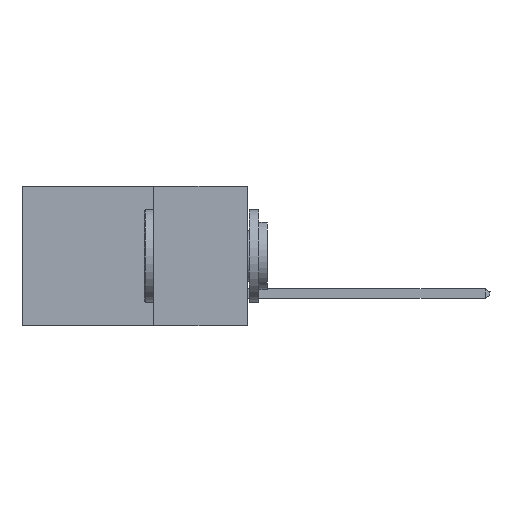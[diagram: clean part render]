
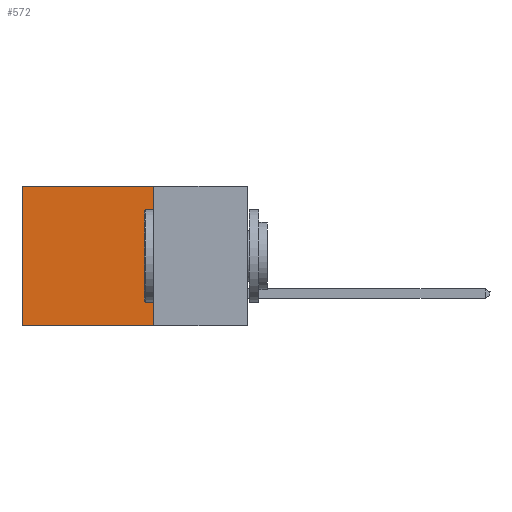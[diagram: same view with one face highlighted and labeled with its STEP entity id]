
A CAD part, left-side view. The second image highlights one B-rep face of the part: STEP entity #572.
In plain terms, the highlighted planar face has unit normal (-1, 0, 0).
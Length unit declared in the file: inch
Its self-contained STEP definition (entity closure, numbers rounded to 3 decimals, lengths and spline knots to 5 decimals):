
#572 = ADVANCED_FACE ( 'NONE', ( #11621 ), #6378, .F. ) ;
#764 = CARTESIAN_POINT ( 'NONE',  ( 0.2615, 0.6, -0.37 ) ) ;
#951 = ORIENTED_EDGE ( 'NONE', *, *, #10089, .F. ) ;
#1567 = VECTOR ( 'NONE', #8770, 39.37008 ) ;
#2288 = LINE ( 'NONE', #6314, #15878 ) ;
#3430 = VERTEX_POINT ( 'NONE', #7115 ) ;
#3524 = DIRECTION ( 'NONE',  ( 0., 1., 0. ) ) ;
#4733 = EDGE_CURVE ( 'NONE', #8559, #3430, #13982, .T. ) ;
#4832 = VERTEX_POINT ( 'NONE', #6330 ) ;
#5613 = VECTOR ( 'NONE', #9853, 39.37008 ) ;
#6314 = CARTESIAN_POINT ( 'NONE',  ( 0.2615, 0.25, -0.37 ) ) ;
#6330 = CARTESIAN_POINT ( 'NONE',  ( 0.2615, 0.25, 0. ) ) ;
#6378 = PLANE ( 'NONE',  #8142 ) ;
#6463 = ORIENTED_EDGE ( 'NONE', *, *, #14785, .T. ) ;
#6838 = CARTESIAN_POINT ( 'NONE',  ( 0.2615, 0.6, 0. ) ) ;
#6924 = ORIENTED_EDGE ( 'NONE', *, *, #4733, .T. ) ;
#7115 = CARTESIAN_POINT ( 'NONE',  ( 0.2615, 0.6, -0.37 ) ) ;
#8142 = AXIS2_PLACEMENT_3D ( 'NONE', #10039, #16994, #13084 ) ;
#8173 = VECTOR ( 'NONE', #14546, 39.37008 ) ;
#8559 = VERTEX_POINT ( 'NONE', #6838 ) ;
#8770 = DIRECTION ( 'NONE',  ( 0., 0., -1. ) ) ;
#9082 = LINE ( 'NONE', #10476, #8173 ) ;
#9273 = VERTEX_POINT ( 'NONE', #14699 ) ;
#9853 = DIRECTION ( 'NONE',  ( 0., 1., 0. ) ) ;
#9882 = ORIENTED_EDGE ( 'NONE', *, *, #14019, .F. ) ;
#10039 = CARTESIAN_POINT ( 'NONE',  ( 0.2615, 0.25, -0.37 ) ) ;
#10089 = EDGE_CURVE ( 'NONE', #4832, #9273, #9082, .T. ) ;
#10476 = CARTESIAN_POINT ( 'NONE',  ( 0.2615, 0.25, -0.37 ) ) ;
#11074 = CARTESIAN_POINT ( 'NONE',  ( 0.2615, 0.25, 0. ) ) ;
#11621 = FACE_OUTER_BOUND ( 'NONE', #16125, .T. ) ;
#13084 = DIRECTION ( 'NONE',  ( 0., 0., -1. ) ) ;
#13761 = LINE ( 'NONE', #11074, #5613 ) ;
#13982 = LINE ( 'NONE', #764, #1567 ) ;
#14019 = EDGE_CURVE ( 'NONE', #9273, #3430, #2288, .T. ) ;
#14546 = DIRECTION ( 'NONE',  ( 0., 0., -1. ) ) ;
#14699 = CARTESIAN_POINT ( 'NONE',  ( 0.2615, 0.25, -0.37 ) ) ;
#14785 = EDGE_CURVE ( 'NONE', #4832, #8559, #13761, .T. ) ;
#15878 = VECTOR ( 'NONE', #3524, 39.37008 ) ;
#16125 = EDGE_LOOP ( 'NONE', ( #6924, #9882, #951, #6463 ) ) ;
#16994 = DIRECTION ( 'NONE',  ( 1., 0., 0. ) ) ;
